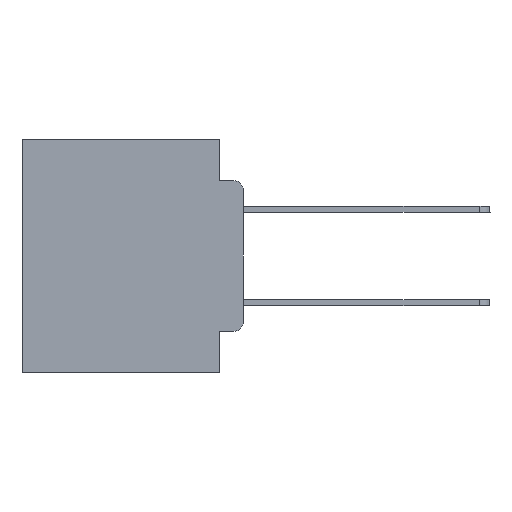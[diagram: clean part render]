
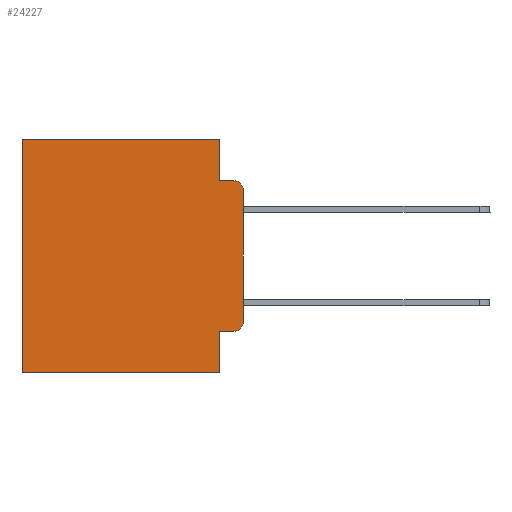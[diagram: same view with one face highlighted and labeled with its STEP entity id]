
A CAD part, left-side view. The second image highlights one B-rep face of the part: STEP entity #24227.
In plain terms, the highlighted planar face has unit normal (-1, 0, 0).
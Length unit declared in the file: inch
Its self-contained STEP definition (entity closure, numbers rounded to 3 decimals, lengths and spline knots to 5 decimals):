
#433 = ORIENTED_EDGE ( 'NONE', *, *, #11035, .T. ) ;
#448 = DIRECTION ( 'NONE',  ( -1., 0., 0. ) ) ;
#470 = VERTEX_POINT ( 'NONE', #8152 ) ;
#576 = VECTOR ( 'NONE', #18485, 39.37008 ) ;
#984 = ORIENTED_EDGE ( 'NONE', *, *, #22762, .T. ) ;
#1072 = DIRECTION ( 'NONE',  ( 0., 0., -1. ) ) ;
#1143 = CARTESIAN_POINT ( 'NONE',  ( 0.298, 0.473, 0. ) ) ;
#1865 = CARTESIAN_POINT ( 'NONE',  ( 0.298, 0., 0. ) ) ;
#2151 = VECTOR ( 'NONE', #5041, 39.37008 ) ;
#2171 = CARTESIAN_POINT ( 'NONE',  ( 0.298, 0.02, -0.0885 ) ) ;
#2212 = DIRECTION ( 'NONE',  ( 0., -1., 0. ) ) ;
#2233 = CIRCLE ( 'NONE', #23709, 0.02 ) ;
#2889 = CIRCLE ( 'NONE', #22494, 0.02 ) ;
#2952 = EDGE_CURVE ( 'NONE', #25914, #16163, #3730, .T. ) ;
#3462 = DIRECTION ( 'NONE',  ( 0., 0., -1. ) ) ;
#3477 = CARTESIAN_POINT ( 'NONE',  ( 0.298, 0.473, -0.5 ) ) ;
#3488 = EDGE_CURVE ( 'NONE', #18381, #26100, #13622, .T. ) ;
#3730 = LINE ( 'NONE', #15067, #2151 ) ;
#4593 = ORIENTED_EDGE ( 'NONE', *, *, #2952, .F. ) ;
#5041 = DIRECTION ( 'NONE',  ( 0., 1., 0. ) ) ;
#5120 = DIRECTION ( 'NONE',  ( 0., -1., 0. ) ) ;
#5122 = VERTEX_POINT ( 'NONE', #2171 ) ;
#5542 = ORIENTED_EDGE ( 'NONE', *, *, #3488, .T. ) ;
#5703 = CARTESIAN_POINT ( 'NONE',  ( 0.298, 0., -0.1085 ) ) ;
#5829 = LINE ( 'NONE', #23643, #23343 ) ;
#6045 = DIRECTION ( 'NONE',  ( 0., 0., -1. ) ) ;
#6717 = CARTESIAN_POINT ( 'NONE',  ( 0.298, 0.051, -0.5 ) ) ;
#6993 = CARTESIAN_POINT ( 'NONE',  ( 0.298, 0.473, 0. ) ) ;
#7261 = CARTESIAN_POINT ( 'NONE',  ( 0.298, 0., 0. ) ) ;
#7353 = DIRECTION ( 'NONE',  ( 0., 0., -1. ) ) ;
#7617 = LINE ( 'NONE', #16145, #19084 ) ;
#7720 = ORIENTED_EDGE ( 'NONE', *, *, #24885, .T. ) ;
#8152 = CARTESIAN_POINT ( 'NONE',  ( 0.298, 0.051, -0.4115 ) ) ;
#8220 = CARTESIAN_POINT ( 'NONE',  ( 0.298, 0.051, -0.0885 ) ) ;
#8345 = DIRECTION ( 'NONE',  ( -1., 0., 0. ) ) ;
#8563 = LINE ( 'NONE', #7261, #20972 ) ;
#9220 = DIRECTION ( 'NONE',  ( 1., 0., 0. ) ) ;
#9400 = CARTESIAN_POINT ( 'NONE',  ( 0.298, 0.051, 0. ) ) ;
#9504 = EDGE_CURVE ( 'NONE', #470, #25914, #18656, .T. ) ;
#10409 = DIRECTION ( 'NONE',  ( 0., 0., -1. ) ) ;
#10463 = DIRECTION ( 'NONE',  ( 0., 0., -1. ) ) ;
#10549 = CARTESIAN_POINT ( 'NONE',  ( 0.298, 0., 0. ) ) ;
#11035 = EDGE_CURVE ( 'NONE', #470, #16884, #5829, .T. ) ;
#11060 = VECTOR ( 'NONE', #23515, 39.37008 ) ;
#11344 = VECTOR ( 'NONE', #3462, 39.37008 ) ;
#11763 = VERTEX_POINT ( 'NONE', #5703 ) ;
#11955 = EDGE_CURVE ( 'NONE', #22477, #5122, #22020, .T. ) ;
#12854 = EDGE_CURVE ( 'NONE', #18381, #22477, #7617, .T. ) ;
#13622 = LINE ( 'NONE', #10549, #576 ) ;
#13823 = CARTESIAN_POINT ( 'NONE',  ( 0.298, 0.051, 0. ) ) ;
#14651 = CARTESIAN_POINT ( 'NONE',  ( 0.298, 0., -0.3915 ) ) ;
#15067 = CARTESIAN_POINT ( 'NONE',  ( 0.298, 0., -0.5 ) ) ;
#15846 = VERTEX_POINT ( 'NONE', #14651 ) ;
#16145 = CARTESIAN_POINT ( 'NONE',  ( 0.298, 0.051, 0. ) ) ;
#16163 = VERTEX_POINT ( 'NONE', #3477 ) ;
#16673 = PLANE ( 'NONE',  #16910 ) ;
#16884 = VERTEX_POINT ( 'NONE', #22372 ) ;
#16910 = AXIS2_PLACEMENT_3D ( 'NONE', #1865, #9220, #1072 ) ;
#17481 = ORIENTED_EDGE ( 'NONE', *, *, #23077, .F. ) ;
#17857 = EDGE_LOOP ( 'NONE', ( #17481, #21097, #24615, #25731, #5542, #7720, #4593, #20081, #433, #984 ) ) ;
#18381 = VERTEX_POINT ( 'NONE', #13823 ) ;
#18485 = DIRECTION ( 'NONE',  ( 0., 1., 0. ) ) ;
#18656 = LINE ( 'NONE', #9400, #11344 ) ;
#19084 = VECTOR ( 'NONE', #6045, 39.37008 ) ;
#20081 = ORIENTED_EDGE ( 'NONE', *, *, #9504, .F. ) ;
#20519 = CARTESIAN_POINT ( 'NONE',  ( 0.298, 0.02, -0.3915 ) ) ;
#20580 = CARTESIAN_POINT ( 'NONE',  ( 0.298, 0.02, -0.1085 ) ) ;
#20922 = FACE_OUTER_BOUND ( 'NONE', #17857, .T. ) ;
#20972 = VECTOR ( 'NONE', #7353, 39.37008 ) ;
#21097 = ORIENTED_EDGE ( 'NONE', *, *, #23392, .T. ) ;
#21215 = LINE ( 'NONE', #1143, #11060 ) ;
#22020 = LINE ( 'NONE', #8220, #24886 ) ;
#22372 = CARTESIAN_POINT ( 'NONE',  ( 0.298, 0.02, -0.4115 ) ) ;
#22477 = VERTEX_POINT ( 'NONE', #25910 ) ;
#22494 = AXIS2_PLACEMENT_3D ( 'NONE', #20519, #8345, #10409 ) ;
#22762 = EDGE_CURVE ( 'NONE', #16884, #15846, #2889, .T. ) ;
#23077 = EDGE_CURVE ( 'NONE', #11763, #15846, #8563, .T. ) ;
#23343 = VECTOR ( 'NONE', #5120, 39.37008 ) ;
#23392 = EDGE_CURVE ( 'NONE', #11763, #5122, #2233, .T. ) ;
#23515 = DIRECTION ( 'NONE',  ( 0., 0., -1. ) ) ;
#23643 = CARTESIAN_POINT ( 'NONE',  ( 0.298, 0.051, -0.4115 ) ) ;
#23709 = AXIS2_PLACEMENT_3D ( 'NONE', #20580, #448, #10463 ) ;
#24227 = ADVANCED_FACE ( 'NONE', ( #20922 ), #16673, .F. ) ;
#24615 = ORIENTED_EDGE ( 'NONE', *, *, #11955, .F. ) ;
#24885 = EDGE_CURVE ( 'NONE', #26100, #16163, #21215, .T. ) ;
#24886 = VECTOR ( 'NONE', #2212, 39.37008 ) ;
#25731 = ORIENTED_EDGE ( 'NONE', *, *, #12854, .F. ) ;
#25910 = CARTESIAN_POINT ( 'NONE',  ( 0.298, 0.051, -0.0885 ) ) ;
#25914 = VERTEX_POINT ( 'NONE', #6717 ) ;
#26100 = VERTEX_POINT ( 'NONE', #6993 ) ;
